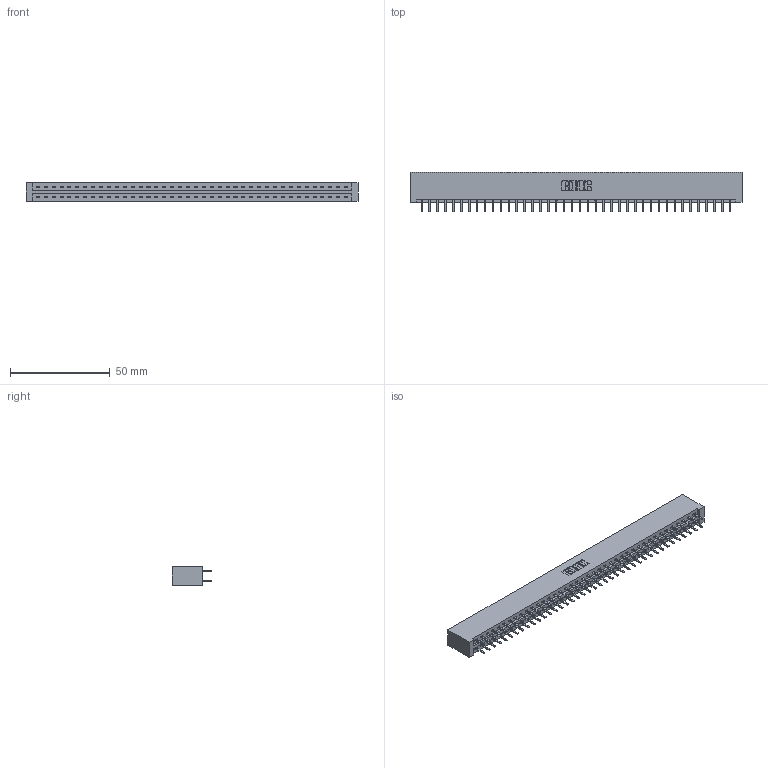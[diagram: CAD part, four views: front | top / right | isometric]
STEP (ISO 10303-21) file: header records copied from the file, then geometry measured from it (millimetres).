
FILE_DESCRIPTION (( 'STEP AP203' ), '1' );
FILE_NAME ('337-080-520-201.STEP', '2018-08-12T17:19:06', ( '' ), ( '' ), 'SwSTEP 2.0', 'SolidWorks 2016', '' );
FILE_SCHEMA (( 'CONFIG_CONTROL_DESIGN' ));
Length unit declared in the file: inch
Products named in the file (3): 337 Part_No Mounting Lugs; 345-292-001_345-293-120; 337-080-520-201
Assembly tree (81 placements, depth 2):
  337-080-520-201
    337 Part_No Mounting Lugs
    345-292-001_345-293-120  x80
Bounding box: 166.37 x 20.02 x 9.4 mm (x, y, z)
Volume: 18232.3 mm3; surface area: 20548.1 mm2
Topology: 81 solids, 81 shells, 4746 faces, 13807 edges, 8990 vertices
Faces by surface type: plane 3266, cylinder 1480
Entity records: 31109 total; most frequent: CARTESIAN_POINT 5254, ORIENTED_EDGE 5178, DIRECTION 4453, EDGE_CURVE 2589, LINE 2465, VECTOR 2465, VERTEX_POINT 1722, AXIS2_PLACEMENT_3D 994
